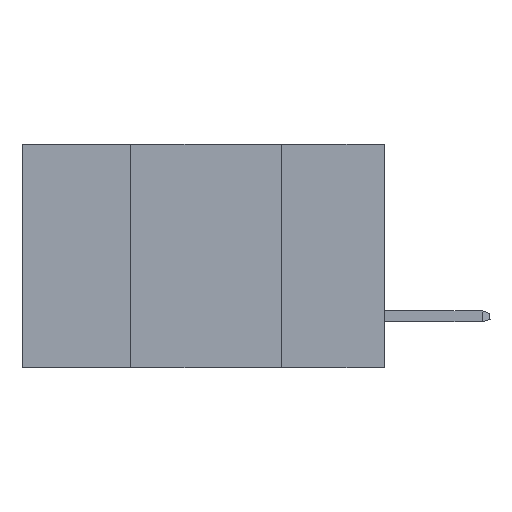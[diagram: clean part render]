
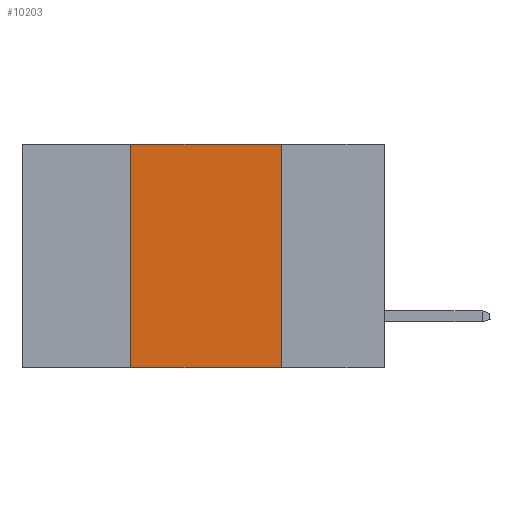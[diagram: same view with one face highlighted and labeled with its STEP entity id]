
A CAD part, left-side view. The second image highlights one B-rep face of the part: STEP entity #10203.
In plain terms, the highlighted planar face has unit normal (-1, 0, 0).
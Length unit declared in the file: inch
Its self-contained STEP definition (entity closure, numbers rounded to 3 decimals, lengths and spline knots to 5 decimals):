
#45 = CARTESIAN_POINT ( 'NONE',  ( 0., 0.17, 0. ) ) ;
#138 = DIRECTION ( 'NONE',  ( 0., 0., -1. ) ) ;
#716 = ORIENTED_EDGE ( 'NONE', *, *, #5553, .F. ) ;
#721 = EDGE_CURVE ( 'NONE', #5825, #4465, #8297, .T. ) ;
#1654 = CARTESIAN_POINT ( 'NONE',  ( 0., 0.6, 0. ) ) ;
#2242 = CARTESIAN_POINT ( 'NONE',  ( 0., 0.42, 0. ) ) ;
#2448 = LINE ( 'NONE', #2242, #14242 ) ;
#2825 = EDGE_CURVE ( 'NONE', #12255, #5825, #8282, .T. ) ;
#3246 = VECTOR ( 'NONE', #9179, 39.37008 ) ;
#4465 = VERTEX_POINT ( 'NONE', #8449 ) ;
#4674 = AXIS2_PLACEMENT_3D ( 'NONE', #1654, #5104, #9799 ) ;
#4687 = CARTESIAN_POINT ( 'NONE',  ( 0., 0.6, 0. ) ) ;
#5104 = DIRECTION ( 'NONE',  ( 1., 0., 0. ) ) ;
#5501 = CARTESIAN_POINT ( 'NONE',  ( 0., 0.42, -0.37 ) ) ;
#5553 = EDGE_CURVE ( 'NONE', #8838, #12255, #2448, .T. ) ;
#5825 = VERTEX_POINT ( 'NONE', #9638 ) ;
#7041 = PLANE ( 'NONE',  #4674 ) ;
#7463 = FACE_OUTER_BOUND ( 'NONE', #8361, .T. ) ;
#7638 = VECTOR ( 'NONE', #11151, 39.37008 ) ;
#7878 = DIRECTION ( 'NONE',  ( 0., 0., 1. ) ) ;
#8282 = LINE ( 'NONE', #4687, #3246 ) ;
#8297 = LINE ( 'NONE', #45, #11835 ) ;
#8361 = EDGE_LOOP ( 'NONE', ( #14252, #14779, #716, #13739 ) ) ;
#8449 = CARTESIAN_POINT ( 'NONE',  ( 0., 0.17, -0.37 ) ) ;
#8838 = VERTEX_POINT ( 'NONE', #5501 ) ;
#8879 = CARTESIAN_POINT ( 'NONE',  ( 0., 0.6, -0.37 ) ) ;
#9179 = DIRECTION ( 'NONE',  ( 0., -1., 0. ) ) ;
#9638 = CARTESIAN_POINT ( 'NONE',  ( 0., 0.17, 0. ) ) ;
#9799 = DIRECTION ( 'NONE',  ( 0., 0., -1. ) ) ;
#10087 = EDGE_CURVE ( 'NONE', #8838, #4465, #10646, .T. ) ;
#10203 = ADVANCED_FACE ( 'NONE', ( #7463 ), #7041, .F. ) ;
#10646 = LINE ( 'NONE', #8879, #7638 ) ;
#11151 = DIRECTION ( 'NONE',  ( 0., -1., 0. ) ) ;
#11835 = VECTOR ( 'NONE', #138, 39.37008 ) ;
#12031 = CARTESIAN_POINT ( 'NONE',  ( 0., 0.42, 0. ) ) ;
#12255 = VERTEX_POINT ( 'NONE', #12031 ) ;
#13739 = ORIENTED_EDGE ( 'NONE', *, *, #10087, .T. ) ;
#14242 = VECTOR ( 'NONE', #7878, 39.37008 ) ;
#14252 = ORIENTED_EDGE ( 'NONE', *, *, #721, .F. ) ;
#14779 = ORIENTED_EDGE ( 'NONE', *, *, #2825, .F. ) ;
